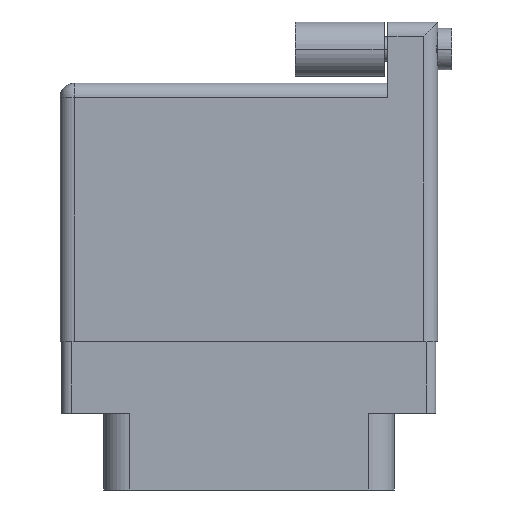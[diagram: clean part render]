
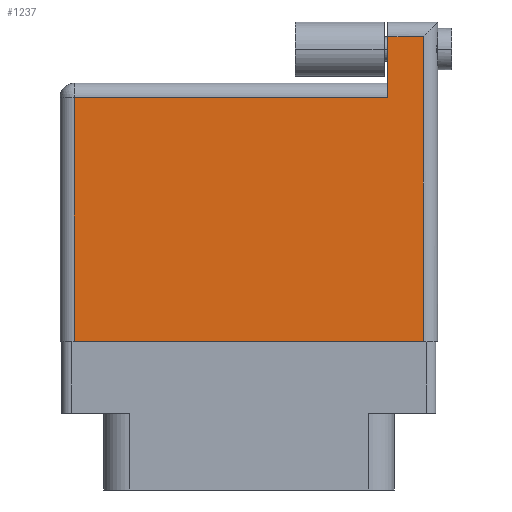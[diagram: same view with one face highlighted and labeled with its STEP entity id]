
A CAD part, front view. The second image highlights one B-rep face of the part: STEP entity #1237.
In plain terms, the highlighted face is planar.
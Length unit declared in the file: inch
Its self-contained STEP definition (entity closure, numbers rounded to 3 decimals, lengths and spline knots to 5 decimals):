
#166 = LINE ( 'NONE', #2792, #18183 ) ;
#326 = ORIENTED_EDGE ( 'NONE', *, *, #3377, .T. ) ;
#722 = VERTEX_POINT ( 'NONE', #7630 ) ;
#1237 = ADVANCED_FACE ( 'NONE', ( #18747 ), #6305, .F. ) ;
#1286 = LINE ( 'NONE', #13955, #12479 ) ;
#1485 = DIRECTION ( 'NONE',  ( 0., -1., 0. ) ) ;
#1487 = ORIENTED_EDGE ( 'NONE', *, *, #14801, .T. ) ;
#1867 = DIRECTION ( 'NONE',  ( 0., 1., 0. ) ) ;
#2195 = VERTEX_POINT ( 'NONE', #7541 ) ;
#2280 = CARTESIAN_POINT ( 'NONE',  ( 1.15, 0.856, 0. ) ) ;
#2792 = CARTESIAN_POINT ( 'NONE',  ( 0.05, 0., 0. ) ) ;
#3377 = EDGE_CURVE ( 'NONE', #2195, #5121, #3797, .T. ) ;
#3797 = LINE ( 'NONE', #18305, #15227 ) ;
#4072 = EDGE_CURVE ( 'NONE', #15072, #722, #1286, .T. ) ;
#4234 = DIRECTION ( 'NONE',  ( -1., 0., 0. ) ) ;
#5121 = VERTEX_POINT ( 'NONE', #2280 ) ;
#5404 = VECTOR ( 'NONE', #4234, 39.37008 ) ;
#5563 = CARTESIAN_POINT ( 'NONE',  ( 0.05, 0.856, 0. ) ) ;
#5757 = DIRECTION ( 'NONE',  ( -1., 0., 0. ) ) ;
#5890 = EDGE_CURVE ( 'NONE', #5121, #16167, #12992, .T. ) ;
#6305 = PLANE ( 'NONE',  #9828 ) ;
#6594 = EDGE_CURVE ( 'NONE', #16167, #15072, #166, .T. ) ;
#6739 = VECTOR ( 'NONE', #5757, 39.37008 ) ;
#7541 = CARTESIAN_POINT ( 'NONE',  ( 1.15, 1.07, 0. ) ) ;
#7630 = CARTESIAN_POINT ( 'NONE',  ( 1.275, 0., 0. ) ) ;
#7666 = LINE ( 'NONE', #10649, #12499 ) ;
#8823 = CARTESIAN_POINT ( 'NONE',  ( 0.05, 0., 0. ) ) ;
#8928 = EDGE_LOOP ( 'NONE', ( #15567, #1487, #10462, #326, #9786, #17831 ) ) ;
#9786 = ORIENTED_EDGE ( 'NONE', *, *, #5890, .T. ) ;
#9828 = AXIS2_PLACEMENT_3D ( 'NONE', #13487, #11043, #15312 ) ;
#9981 = CARTESIAN_POINT ( 'NONE',  ( 1.275, 1.07, 0. ) ) ;
#10207 = CARTESIAN_POINT ( 'NONE',  ( 0., 1.07, 0. ) ) ;
#10462 = ORIENTED_EDGE ( 'NONE', *, *, #14522, .T. ) ;
#10649 = CARTESIAN_POINT ( 'NONE',  ( 1.275, 1.12, 0. ) ) ;
#11043 = DIRECTION ( 'NONE',  ( 0., 0., -1. ) ) ;
#11247 = VERTEX_POINT ( 'NONE', #9981 ) ;
#11818 = LINE ( 'NONE', #10207, #6739 ) ;
#12479 = VECTOR ( 'NONE', #18473, 39.37008 ) ;
#12499 = VECTOR ( 'NONE', #1867, 39.37008 ) ;
#12882 = CARTESIAN_POINT ( 'NONE',  ( 0., 0.856, 0. ) ) ;
#12992 = LINE ( 'NONE', #12882, #5404 ) ;
#13487 = CARTESIAN_POINT ( 'NONE',  ( 0., 0.906, 0. ) ) ;
#13955 = CARTESIAN_POINT ( 'NONE',  ( 0., 0., 0. ) ) ;
#13977 = DIRECTION ( 'NONE',  ( 0., -1., 0. ) ) ;
#14522 = EDGE_CURVE ( 'NONE', #11247, #2195, #11818, .T. ) ;
#14801 = EDGE_CURVE ( 'NONE', #722, #11247, #7666, .T. ) ;
#15072 = VERTEX_POINT ( 'NONE', #8823 ) ;
#15227 = VECTOR ( 'NONE', #13977, 39.37008 ) ;
#15312 = DIRECTION ( 'NONE',  ( -1., 0., 0. ) ) ;
#15567 = ORIENTED_EDGE ( 'NONE', *, *, #4072, .T. ) ;
#16167 = VERTEX_POINT ( 'NONE', #5563 ) ;
#17831 = ORIENTED_EDGE ( 'NONE', *, *, #6594, .T. ) ;
#18183 = VECTOR ( 'NONE', #1485, 39.37008 ) ;
#18305 = CARTESIAN_POINT ( 'NONE',  ( 1.15, 1.12, 0. ) ) ;
#18473 = DIRECTION ( 'NONE',  ( 1., 0., 0. ) ) ;
#18747 = FACE_OUTER_BOUND ( 'NONE', #8928, .T. ) ;
